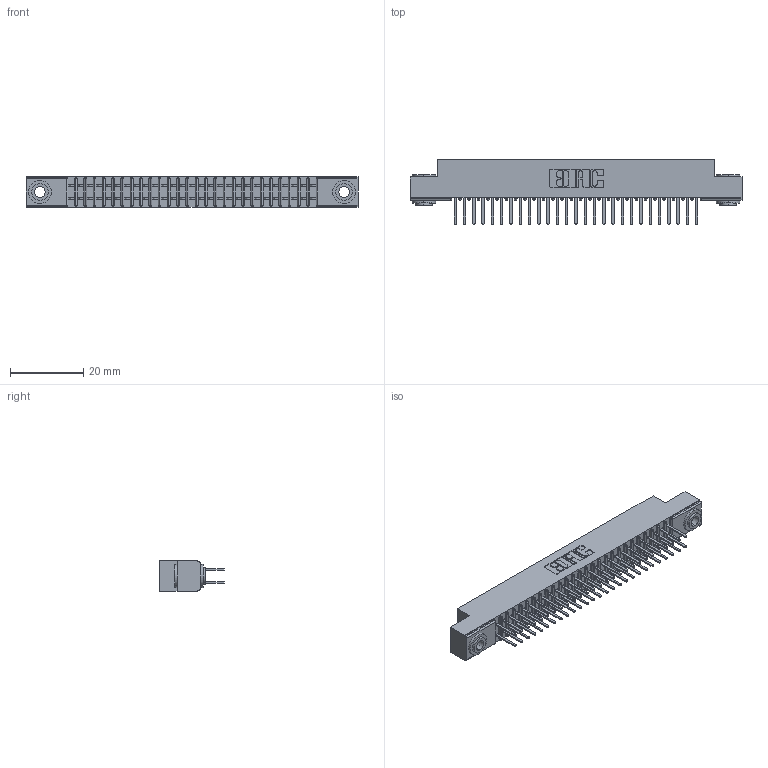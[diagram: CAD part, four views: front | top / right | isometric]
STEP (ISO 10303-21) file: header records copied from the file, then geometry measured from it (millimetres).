
FILE_DESCRIPTION (( 'STEP AP203' ), '1' );
FILE_NAME ('341-054-521-203.STEP', '2018-08-07T14:11:30', ( '' ), ( '' ), 'SwSTEP 2.0', 'SolidWorks 2016', '' );
FILE_SCHEMA (( 'CONFIG_CONTROL_DESIGN' ));
Length unit declared in the file: inch
Products named in the file (4): 345-250-002_345-250-002-102; 341-054-521-203; 341 Part_.156 (3.96) Dia Mounting Holes; 341-292-001_341-292-121
Assembly tree (57 placements, depth 2):
  341-054-521-203
    341 Part_.156 (3.96) Dia Mounting Holes
    341-292-001_341-292-121  x54
    345-250-002_345-250-002-102  x2
Bounding box: 90.81 x 17.7 x 8.38 mm (x, y, z)
Volume: 5198.2 mm3; surface area: 11603.5 mm2
Topology: 57 solids, 57 shells, 3732 faces, 10769 edges, 6974 vertices
Faces by surface type: plane 2252, cylinder 1364, sphere 56, torus 52, cone 8
Entity records: 35739 total; most frequent: CARTESIAN_POINT 5922, ORIENTED_EDGE 5874, DIRECTION 5773, EDGE_CURVE 2937, LINE 2347, VECTOR 2347, VERTEX_POINT 1862, AXIS2_PLACEMENT_3D 1713
